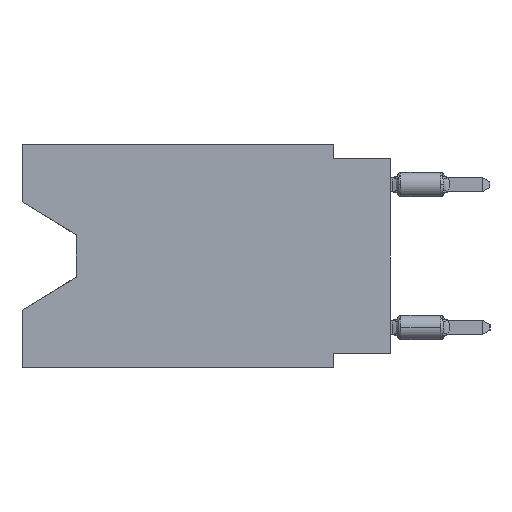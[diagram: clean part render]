
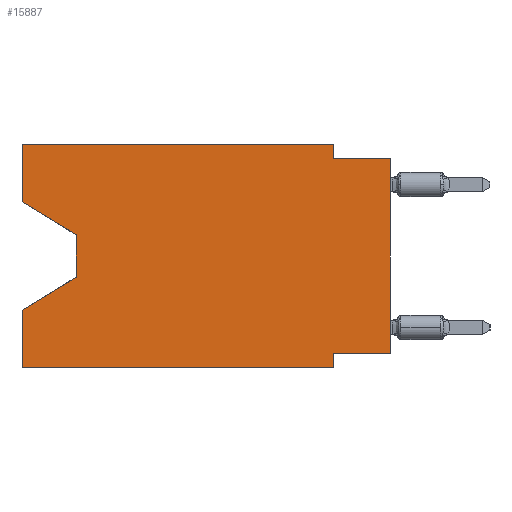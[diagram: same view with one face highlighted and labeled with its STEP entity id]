
A CAD part, left-side view. The second image highlights one B-rep face of the part: STEP entity #15887.
In plain terms, the highlighted planar face has unit normal (-1, 0, 0).
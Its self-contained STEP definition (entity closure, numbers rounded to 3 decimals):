
#424 = EDGE_CURVE ( 'NONE', #8348, #8085, #21558, .T. ) ;
#465 = DIRECTION ( 'NONE',  ( 0., -1., 0. ) ) ;
#638 = VERTEX_POINT ( 'NONE', #43499 ) ;
#706 = ORIENTED_EDGE ( 'NONE', *, *, #12363, .F. ) ;
#868 = EDGE_CURVE ( 'NONE', #40841, #38086, #41027, .T. ) ;
#950 = DIRECTION ( 'NONE',  ( 0., 0., 1. ) ) ;
#976 = EDGE_CURVE ( 'NONE', #38086, #25055, #22374, .T. ) ;
#1065 = CARTESIAN_POINT ( 'NONE',  ( 0., 16.383, 0. ) ) ;
#1074 = CARTESIAN_POINT ( 'NONE',  ( 0., 2.54, -0.635 ) ) ;
#1878 = DIRECTION ( 'NONE',  ( 0., 0., 1. ) ) ;
#3522 = VECTOR ( 'NONE', #40250, 1000. ) ;
#4507 = CARTESIAN_POINT ( 'NONE',  ( 0., 2.54, -9.906 ) ) ;
#4546 = VECTOR ( 'NONE', #4607, 1000. ) ;
#4607 = DIRECTION ( 'NONE',  ( 0., 0., -1. ) ) ;
#4942 = EDGE_CURVE ( 'NONE', #8348, #41086, #31988, .T. ) ;
#4999 = VECTOR ( 'NONE', #24776, 1000. ) ;
#5647 = CARTESIAN_POINT ( 'NONE',  ( 0., 16.383, 0. ) ) ;
#5969 = EDGE_LOOP ( 'NONE', ( #24709, #12868, #42714, #27763, #24871, #35679, #6797, #12450, #25166, #706, #38319, #33267 ) ) ;
#6018 = VECTOR ( 'NONE', #950, 1000. ) ;
#6092 = DIRECTION ( 'NONE',  ( 0., 0., -1. ) ) ;
#6797 = ORIENTED_EDGE ( 'NONE', *, *, #868, .F. ) ;
#6857 = EDGE_CURVE ( 'NONE', #11529, #9823, #24595, .T. ) ;
#8085 = VERTEX_POINT ( 'NONE', #37074 ) ;
#8348 = VERTEX_POINT ( 'NONE', #15751 ) ;
#8709 = VECTOR ( 'NONE', #27685, 1000. ) ;
#9394 = PLANE ( 'NONE',  #29917 ) ;
#9823 = VERTEX_POINT ( 'NONE', #31669 ) ;
#9886 = CARTESIAN_POINT ( 'NONE',  ( 0., 13.97, -5.893 ) ) ;
#10449 = LINE ( 'NONE', #17301, #16933 ) ;
#10525 = EDGE_CURVE ( 'NONE', #40841, #9823, #21858, .T. ) ;
#10669 = CARTESIAN_POINT ( 'NONE',  ( 0., 0., -9.271 ) ) ;
#11292 = LINE ( 'NONE', #21693, #4999 ) ;
#11529 = VERTEX_POINT ( 'NONE', #1074 ) ;
#11914 = CARTESIAN_POINT ( 'NONE',  ( 0., 0., 0. ) ) ;
#12192 = DIRECTION ( 'NONE',  ( 0., 0., -1. ) ) ;
#12363 = EDGE_CURVE ( 'NONE', #26969, #11529, #11292, .T. ) ;
#12450 = ORIENTED_EDGE ( 'NONE', *, *, #10525, .T. ) ;
#12868 = ORIENTED_EDGE ( 'NONE', *, *, #24235, .T. ) ;
#14189 = LINE ( 'NONE', #28130, #8709 ) ;
#14561 = LINE ( 'NONE', #24951, #4546 ) ;
#15064 = CARTESIAN_POINT ( 'NONE',  ( 0., 2.54, -9.906 ) ) ;
#15751 = CARTESIAN_POINT ( 'NONE',  ( 0., 16.383, -2.546 ) ) ;
#15887 = ADVANCED_FACE ( 'NONE', ( #42629 ), #9394, .F. ) ;
#16460 = DIRECTION ( 'NONE',  ( 1., 0., 0. ) ) ;
#16586 = VERTEX_POINT ( 'NONE', #9886 ) ;
#16933 = VECTOR ( 'NONE', #465, 1000. ) ;
#17301 = CARTESIAN_POINT ( 'NONE',  ( 0., 16.383, 0. ) ) ;
#18190 = EDGE_CURVE ( 'NONE', #43674, #25055, #29386, .T. ) ;
#18242 = DIRECTION ( 'NONE',  ( 0., -0.855, -0.519 ) ) ;
#19260 = VECTOR ( 'NONE', #41242, 1000. ) ;
#19395 = CARTESIAN_POINT ( 'NONE',  ( 0., 2.54, -9.271 ) ) ;
#19750 = VECTOR ( 'NONE', #12192, 1000. ) ;
#20905 = LINE ( 'NONE', #31289, #6018 ) ;
#21558 = LINE ( 'NONE', #42174, #29600 ) ;
#21693 = CARTESIAN_POINT ( 'NONE',  ( 0., 2.54, 0. ) ) ;
#21858 = LINE ( 'NONE', #11914, #3522 ) ;
#22374 = LINE ( 'NONE', #15064, #19750 ) ;
#22889 = CARTESIAN_POINT ( 'NONE',  ( 0., 16.383, 0. ) ) ;
#24235 = EDGE_CURVE ( 'NONE', #8085, #16586, #14561, .T. ) ;
#24534 = VECTOR ( 'NONE', #1878, 1000. ) ;
#24595 = LINE ( 'NONE', #27479, #19260 ) ;
#24709 = ORIENTED_EDGE ( 'NONE', *, *, #424, .T. ) ;
#24776 = DIRECTION ( 'NONE',  ( 0., 0., -1. ) ) ;
#24871 = ORIENTED_EDGE ( 'NONE', *, *, #18190, .T. ) ;
#24951 = CARTESIAN_POINT ( 'NONE',  ( 0., 13.97, -4.013 ) ) ;
#25027 = EDGE_CURVE ( 'NONE', #43674, #638, #20905, .T. ) ;
#25055 = VERTEX_POINT ( 'NONE', #4507 ) ;
#25166 = ORIENTED_EDGE ( 'NONE', *, *, #6857, .F. ) ;
#25397 = CARTESIAN_POINT ( 'NONE',  ( 0., 16.383, -9.906 ) ) ;
#25900 = CARTESIAN_POINT ( 'NONE',  ( 0., 0., -9.271 ) ) ;
#26728 = EDGE_CURVE ( 'NONE', #16586, #638, #14189, .T. ) ;
#26969 = VERTEX_POINT ( 'NONE', #40762 ) ;
#27479 = CARTESIAN_POINT ( 'NONE',  ( 0., 0., -0.635 ) ) ;
#27685 = DIRECTION ( 'NONE',  ( 0., 0.855, -0.519 ) ) ;
#27763 = ORIENTED_EDGE ( 'NONE', *, *, #25027, .F. ) ;
#28130 = CARTESIAN_POINT ( 'NONE',  ( 0., 13.97, -5.893 ) ) ;
#29386 = LINE ( 'NONE', #25397, #33311 ) ;
#29600 = VECTOR ( 'NONE', #18242, 1000. ) ;
#29917 = AXIS2_PLACEMENT_3D ( 'NONE', #22889, #16460, #6092 ) ;
#31289 = CARTESIAN_POINT ( 'NONE',  ( 0., 16.383, 0. ) ) ;
#31669 = CARTESIAN_POINT ( 'NONE',  ( 0., 0., -0.635 ) ) ;
#31745 = VECTOR ( 'NONE', #41474, 1000. ) ;
#31988 = LINE ( 'NONE', #5647, #24534 ) ;
#33267 = ORIENTED_EDGE ( 'NONE', *, *, #4942, .F. ) ;
#33311 = VECTOR ( 'NONE', #35592, 1000. ) ;
#35592 = DIRECTION ( 'NONE',  ( 0., -1., 0. ) ) ;
#35679 = ORIENTED_EDGE ( 'NONE', *, *, #976, .F. ) ;
#37074 = CARTESIAN_POINT ( 'NONE',  ( 0., 13.97, -4.013 ) ) ;
#38086 = VERTEX_POINT ( 'NONE', #19395 ) ;
#38319 = ORIENTED_EDGE ( 'NONE', *, *, #40705, .F. ) ;
#40063 = CARTESIAN_POINT ( 'NONE',  ( 0., 16.383, -9.906 ) ) ;
#40250 = DIRECTION ( 'NONE',  ( 0., 0., 1. ) ) ;
#40705 = EDGE_CURVE ( 'NONE', #41086, #26969, #10449, .T. ) ;
#40762 = CARTESIAN_POINT ( 'NONE',  ( 0., 2.54, 0. ) ) ;
#40841 = VERTEX_POINT ( 'NONE', #25900 ) ;
#41027 = LINE ( 'NONE', #10669, #31745 ) ;
#41086 = VERTEX_POINT ( 'NONE', #1065 ) ;
#41242 = DIRECTION ( 'NONE',  ( 0., -1., 0. ) ) ;
#41474 = DIRECTION ( 'NONE',  ( 0., 1., 0. ) ) ;
#42174 = CARTESIAN_POINT ( 'NONE',  ( 0., 16.383, -2.546 ) ) ;
#42629 = FACE_OUTER_BOUND ( 'NONE', #5969, .T. ) ;
#42714 = ORIENTED_EDGE ( 'NONE', *, *, #26728, .T. ) ;
#43499 = CARTESIAN_POINT ( 'NONE',  ( 0., 16.383, -7.36 ) ) ;
#43674 = VERTEX_POINT ( 'NONE', #40063 ) ;
